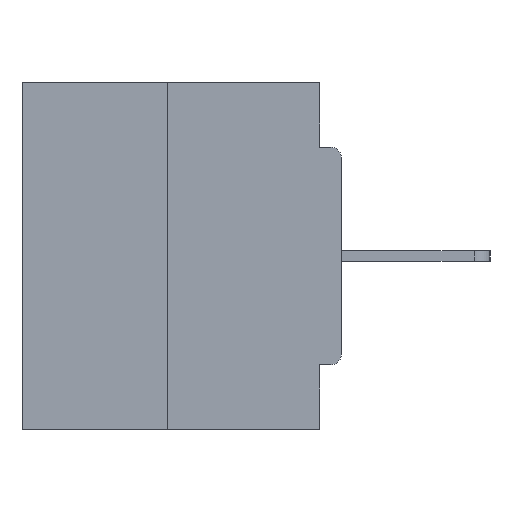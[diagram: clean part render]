
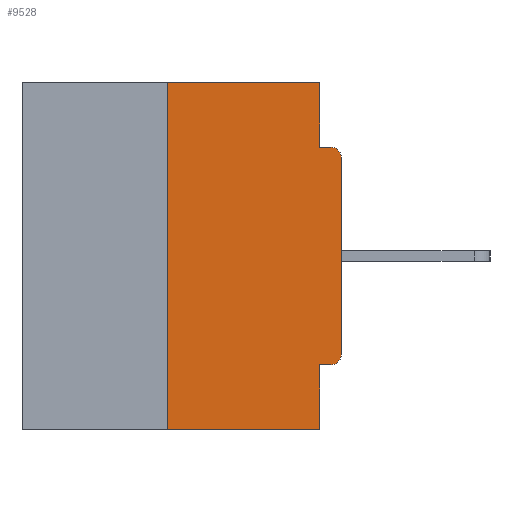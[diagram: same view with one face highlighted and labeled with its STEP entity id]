
A CAD part, left-side view. The second image highlights one B-rep face of the part: STEP entity #9528.
In plain terms, the highlighted planar face has unit normal (-1, 0, 0).
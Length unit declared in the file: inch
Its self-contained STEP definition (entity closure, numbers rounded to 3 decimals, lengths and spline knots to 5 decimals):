
#169 = CARTESIAN_POINT ( 'NONE',  ( 0., 0.25, 0. ) ) ;
#395 = DIRECTION ( 'NONE',  ( 0., 0., -1. ) ) ;
#459 = AXIS2_PLACEMENT_3D ( 'NONE', #25907, #28668, #23744 ) ;
#767 = CARTESIAN_POINT ( 'NONE',  ( 0., 0., -0.0935 ) ) ;
#1391 = CARTESIAN_POINT ( 'NONE',  ( 0., 0.031, 0. ) ) ;
#1434 = LINE ( 'NONE', #28409, #14819 ) ;
#1487 = ORIENTED_EDGE ( 'NONE', *, *, #28104, .F. ) ;
#1938 = VECTOR ( 'NONE', #13234, 39.37008 ) ;
#2590 = CARTESIAN_POINT ( 'NONE',  ( 0., 0.015, -0.4065 ) ) ;
#2817 = LINE ( 'NONE', #13996, #19968 ) ;
#3074 = LINE ( 'NONE', #767, #6719 ) ;
#3292 = VERTEX_POINT ( 'NONE', #18886 ) ;
#3965 = CARTESIAN_POINT ( 'NONE',  ( 0., 0.031, -0.5 ) ) ;
#4465 = EDGE_CURVE ( 'NONE', #27661, #27004, #7119, .T. ) ;
#4653 = VERTEX_POINT ( 'NONE', #17284 ) ;
#4893 = LINE ( 'NONE', #5028, #22615 ) ;
#5028 = CARTESIAN_POINT ( 'NONE',  ( 0., 0., -0.4065 ) ) ;
#5526 = ORIENTED_EDGE ( 'NONE', *, *, #27374, .F. ) ;
#5752 = EDGE_CURVE ( 'NONE', #27004, #9382, #23237, .T. ) ;
#5862 = ORIENTED_EDGE ( 'NONE', *, *, #5752, .F. ) ;
#6041 = PLANE ( 'NONE',  #459 ) ;
#6719 = VECTOR ( 'NONE', #23108, 39.37008 ) ;
#6921 = DIRECTION ( 'NONE',  ( 0., 1., 0. ) ) ;
#7119 = LINE ( 'NONE', #169, #1938 ) ;
#7240 = CARTESIAN_POINT ( 'NONE',  ( 0., 0.25, 0. ) ) ;
#7317 = VECTOR ( 'NONE', #12052, 39.37008 ) ;
#7506 = EDGE_CURVE ( 'NONE', #27661, #12208, #1434, .T. ) ;
#8246 = EDGE_CURVE ( 'NONE', #3292, #4653, #2817, .T. ) ;
#8296 = VECTOR ( 'NONE', #28481, 39.37008 ) ;
#8835 = ORIENTED_EDGE ( 'NONE', *, *, #15495, .F. ) ;
#8907 = ORIENTED_EDGE ( 'NONE', *, *, #8246, .T. ) ;
#9041 = CARTESIAN_POINT ( 'NONE',  ( 0., 0.015, -0.0935 ) ) ;
#9265 = EDGE_CURVE ( 'NONE', #16345, #3292, #18091, .T. ) ;
#9382 = VERTEX_POINT ( 'NONE', #1391 ) ;
#9528 = ADVANCED_FACE ( 'NONE', ( #22139 ), #6041, .F. ) ;
#10175 = CARTESIAN_POINT ( 'NONE',  ( 0., 0.46, 0. ) ) ;
#10594 = ORIENTED_EDGE ( 'NONE', *, *, #4465, .F. ) ;
#11313 = VERTEX_POINT ( 'NONE', #9041 ) ;
#12052 = DIRECTION ( 'NONE',  ( 0., -1., 0. ) ) ;
#12208 = VERTEX_POINT ( 'NONE', #22179 ) ;
#12379 = CARTESIAN_POINT ( 'NONE',  ( 0., 0.015, -0.1085 ) ) ;
#12814 = DIRECTION ( 'NONE',  ( 0., 0., -1. ) ) ;
#13207 = ORIENTED_EDGE ( 'NONE', *, *, #21417, .T. ) ;
#13234 = DIRECTION ( 'NONE',  ( 0., 0., 1. ) ) ;
#13996 = CARTESIAN_POINT ( 'NONE',  ( 0., 0., 0. ) ) ;
#14593 = EDGE_LOOP ( 'NONE', ( #5862, #10594, #23532, #1487, #5526, #27096, #8907, #13207, #8835, #28365 ) ) ;
#14819 = VECTOR ( 'NONE', #26382, 39.37008 ) ;
#15495 = EDGE_CURVE ( 'NONE', #28182, #11313, #3074, .T. ) ;
#16210 = DIRECTION ( 'NONE',  ( 0., 0., -1. ) ) ;
#16345 = VERTEX_POINT ( 'NONE', #2590 ) ;
#17284 = CARTESIAN_POINT ( 'NONE',  ( 0., 0., -0.1085 ) ) ;
#18032 = VECTOR ( 'NONE', #12814, 39.37008 ) ;
#18091 = CIRCLE ( 'NONE', #22697, 0.015 ) ;
#18886 = CARTESIAN_POINT ( 'NONE',  ( 0., 0., -0.3915 ) ) ;
#19644 = CARTESIAN_POINT ( 'NONE',  ( 0., 0.031, 0. ) ) ;
#19968 = VECTOR ( 'NONE', #22845, 39.37008 ) ;
#20273 = DIRECTION ( 'NONE',  ( -1., 0., 0. ) ) ;
#21310 = CARTESIAN_POINT ( 'NONE',  ( 0., 0.031, -0.4065 ) ) ;
#21417 = EDGE_CURVE ( 'NONE', #4653, #11313, #28426, .T. ) ;
#22139 = FACE_OUTER_BOUND ( 'NONE', #14593, .T. ) ;
#22179 = CARTESIAN_POINT ( 'NONE',  ( 0., 0.031, -0.5 ) ) ;
#22308 = DIRECTION ( 'NONE',  ( -1., 0., 0. ) ) ;
#22321 = VERTEX_POINT ( 'NONE', #21310 ) ;
#22615 = VECTOR ( 'NONE', #6921, 39.37008 ) ;
#22697 = AXIS2_PLACEMENT_3D ( 'NONE', #27216, #22308, #16210 ) ;
#22845 = DIRECTION ( 'NONE',  ( 0., 0., 1. ) ) ;
#22871 = AXIS2_PLACEMENT_3D ( 'NONE', #12379, #20273, #395 ) ;
#23108 = DIRECTION ( 'NONE',  ( 0., -1., 0. ) ) ;
#23237 = LINE ( 'NONE', #10175, #7317 ) ;
#23532 = ORIENTED_EDGE ( 'NONE', *, *, #7506, .T. ) ;
#23708 = LINE ( 'NONE', #3965, #18032 ) ;
#23744 = DIRECTION ( 'NONE',  ( 0., 0., -1. ) ) ;
#25907 = CARTESIAN_POINT ( 'NONE',  ( 0., 0.46, 0. ) ) ;
#26049 = CARTESIAN_POINT ( 'NONE',  ( 0., 0.25, -0.5 ) ) ;
#26382 = DIRECTION ( 'NONE',  ( 0., -1., 0. ) ) ;
#26442 = LINE ( 'NONE', #19644, #8296 ) ;
#26732 = CARTESIAN_POINT ( 'NONE',  ( 0., 0.031, -0.0935 ) ) ;
#27004 = VERTEX_POINT ( 'NONE', #7240 ) ;
#27096 = ORIENTED_EDGE ( 'NONE', *, *, #9265, .T. ) ;
#27216 = CARTESIAN_POINT ( 'NONE',  ( 0., 0.015, -0.3915 ) ) ;
#27374 = EDGE_CURVE ( 'NONE', #16345, #22321, #4893, .T. ) ;
#27661 = VERTEX_POINT ( 'NONE', #26049 ) ;
#28104 = EDGE_CURVE ( 'NONE', #22321, #12208, #23708, .T. ) ;
#28182 = VERTEX_POINT ( 'NONE', #26732 ) ;
#28215 = EDGE_CURVE ( 'NONE', #9382, #28182, #26442, .T. ) ;
#28365 = ORIENTED_EDGE ( 'NONE', *, *, #28215, .F. ) ;
#28409 = CARTESIAN_POINT ( 'NONE',  ( 0., 0.46, -0.5 ) ) ;
#28426 = CIRCLE ( 'NONE', #22871, 0.015 ) ;
#28481 = DIRECTION ( 'NONE',  ( 0., 0., -1. ) ) ;
#28668 = DIRECTION ( 'NONE',  ( 1., 0., 0. ) ) ;
